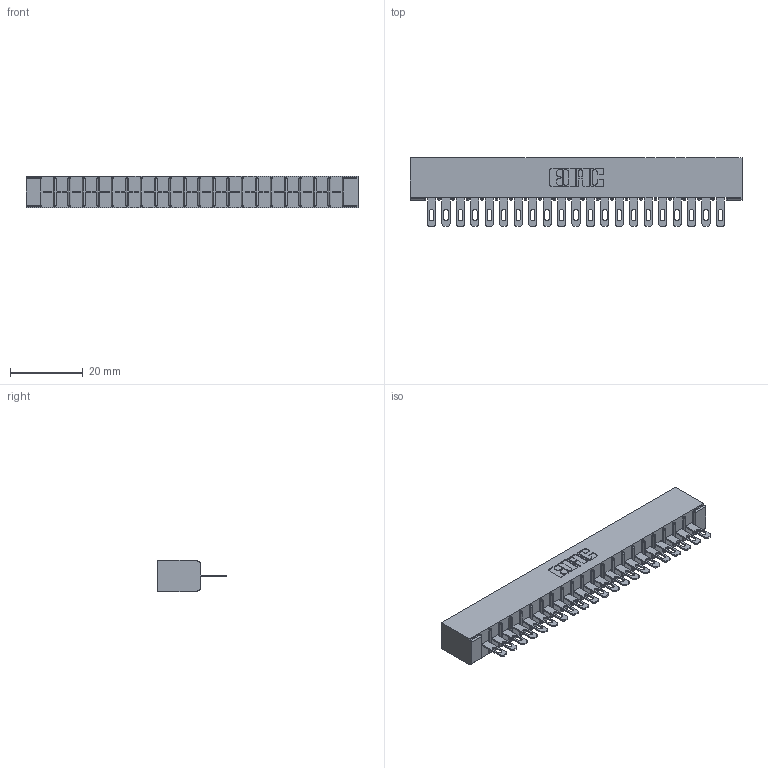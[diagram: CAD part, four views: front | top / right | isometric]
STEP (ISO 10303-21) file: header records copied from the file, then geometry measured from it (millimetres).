
FILE_DESCRIPTION (( 'STEP AP203' ), '1' );
FILE_NAME ('316-021-400-101.STEP', '2020-09-22T19:48:58', ( '' ), ( '' ), 'SwSTEP 2.0', 'SolidWorks 2020', '' );
FILE_SCHEMA (( 'CONFIG_CONTROL_DESIGN' ));
Length unit declared in the file: inch
Products named in the file (3): 306 Part_No Mounting; 306-290-001_100; 316-021-400-101
Assembly tree (22 placements, depth 2):
  316-021-400-101
    306 Part_No Mounting
    306-290-001_100  x21
Bounding box: 91.08 x 18.87 x 8.71 mm (x, y, z)
Volume: 6573.2 mm3; surface area: 10270.4 mm2
Topology: 22 solids, 22 shells, 1704 faces, 4807 edges, 3090 vertices
Faces by surface type: plane 1114, cylinder 506, sphere 84
Entity records: 22190 total; most frequent: CARTESIAN_POINT 3722, ORIENTED_EDGE 3686, DIRECTION 3673, EDGE_CURVE 1843, LINE 1431, VECTOR 1431, VERTEX_POINT 1170, AXIS2_PLACEMENT_3D 1121
